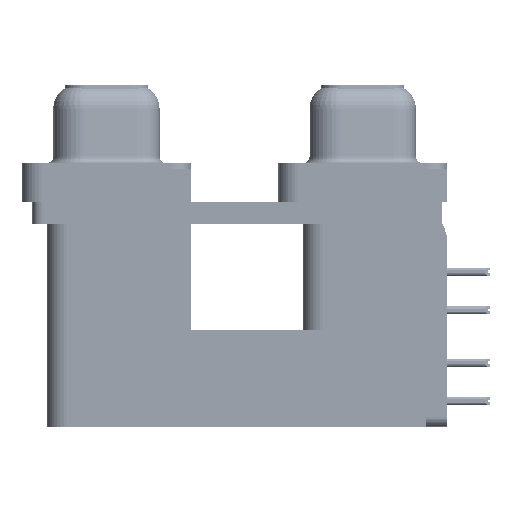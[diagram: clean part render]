
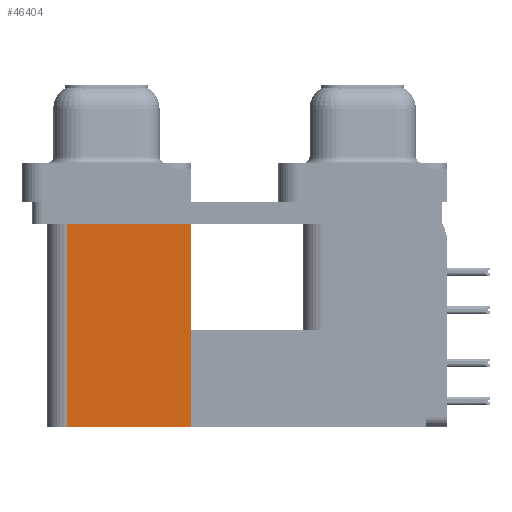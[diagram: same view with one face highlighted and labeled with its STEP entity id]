
A CAD part, left-side view. The second image highlights one B-rep face of the part: STEP entity #46404.
In plain terms, the highlighted planar face has unit normal (-1, 0, 0).
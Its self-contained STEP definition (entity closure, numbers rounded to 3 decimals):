
#4809 = ORIENTED_EDGE ( 'NONE', *, *, #53689, .T. ) ;
#5235 = EDGE_CURVE ( 'NONE', #27249, #57888, #6311, .T. ) ;
#5357 = LINE ( 'NONE', #51837, #52677 ) ;
#6010 = DIRECTION ( 'NONE',  ( 1., 0., 0. ) ) ;
#6311 = LINE ( 'NONE', #52482, #31090 ) ;
#6318 = DIRECTION ( 'NONE',  ( 0., 1., 0. ) ) ;
#7401 = CARTESIAN_POINT ( 'NONE',  ( 3.7, 21.975, -2.5 ) ) ;
#9141 = AXIS2_PLACEMENT_3D ( 'NONE', #47898, #6010, #6318 ) ;
#10344 = DIRECTION ( 'NONE',  ( 0., 0., 1. ) ) ;
#12376 = EDGE_CURVE ( 'NONE', #28154, #57888, #53148, .T. ) ;
#12649 = DIRECTION ( 'NONE',  ( 0., 0., 1. ) ) ;
#14274 = PLANE ( 'NONE',  #9141 ) ;
#25513 = LINE ( 'NONE', #26119, #34043 ) ;
#26119 = CARTESIAN_POINT ( 'NONE',  ( 3.7, 12.775, -19.2 ) ) ;
#27249 = VERTEX_POINT ( 'NONE', #41799 ) ;
#28154 = VERTEX_POINT ( 'NONE', #49574 ) ;
#29243 = DIRECTION ( 'NONE',  ( 0., 1., 0. ) ) ;
#31090 = VECTOR ( 'NONE', #29243, 1000. ) ;
#31576 = VERTEX_POINT ( 'NONE', #59243 ) ;
#34043 = VECTOR ( 'NONE', #12649, 1000. ) ;
#34141 = FACE_OUTER_BOUND ( 'NONE', #55916, .T. ) ;
#38191 = ORIENTED_EDGE ( 'NONE', *, *, #5235, .T. ) ;
#38374 = DIRECTION ( 'NONE',  ( 0., 1., 0. ) ) ;
#39783 = ORIENTED_EDGE ( 'NONE', *, *, #55169, .F. ) ;
#41799 = CARTESIAN_POINT ( 'NONE',  ( 3.7, 12.775, -2.5 ) ) ;
#46404 = ADVANCED_FACE ( 'NONE', ( #34141 ), #14274, .F. ) ;
#47898 = CARTESIAN_POINT ( 'NONE',  ( 3.7, 12.775, -19.2 ) ) ;
#49574 = CARTESIAN_POINT ( 'NONE',  ( 3.7, 21.975, -19.2 ) ) ;
#51837 = CARTESIAN_POINT ( 'NONE',  ( 3.7, 12.775, -19.2 ) ) ;
#52482 = CARTESIAN_POINT ( 'NONE',  ( 3.7, 12.775, -2.5 ) ) ;
#52677 = VECTOR ( 'NONE', #38374, 1000. ) ;
#53148 = LINE ( 'NONE', #57721, #53374 ) ;
#53374 = VECTOR ( 'NONE', #10344, 1000. ) ;
#53689 = EDGE_CURVE ( 'NONE', #31576, #27249, #25513, .T. ) ;
#54014 = ORIENTED_EDGE ( 'NONE', *, *, #12376, .F. ) ;
#55169 = EDGE_CURVE ( 'NONE', #31576, #28154, #5357, .T. ) ;
#55916 = EDGE_LOOP ( 'NONE', ( #38191, #54014, #39783, #4809 ) ) ;
#57721 = CARTESIAN_POINT ( 'NONE',  ( 3.7, 21.975, -19.2 ) ) ;
#57888 = VERTEX_POINT ( 'NONE', #7401 ) ;
#59243 = CARTESIAN_POINT ( 'NONE',  ( 3.7, 12.775, -19.2 ) ) ;
